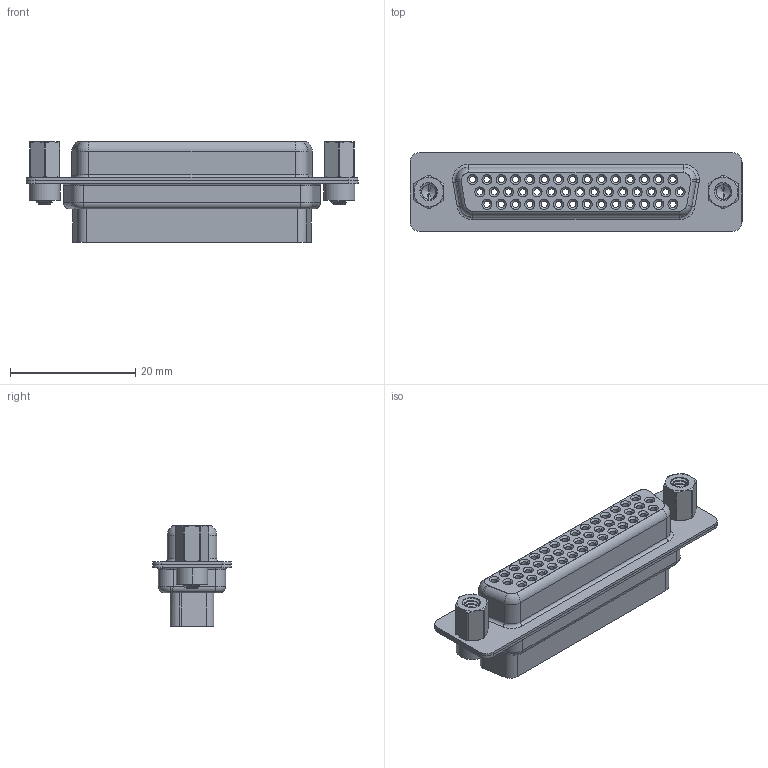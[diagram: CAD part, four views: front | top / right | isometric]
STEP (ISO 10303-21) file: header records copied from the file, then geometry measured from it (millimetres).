
FILE_DESCRIPTION (( 'STEP AP203' ), '1' );
FILE_NAME ('638-044-010-043.STEP', '2020-07-18T16:41:01', ( '' ), ( '' ), 'SwSTEP 2.0', 'SolidWorks 2020', '' );
FILE_SCHEMA (( 'CONFIG_CONTROL_DESIGN' ));
Length unit declared in the file: millimetre
Products named in the file (6): 638-044-010-043; 638 Housing_44 Contacts HP; 638 Shell Rear_44 Contacts; 638 Shell Front_44 Contacts; 638 4-40 Threaded Rivet; 638 4-40 Hex Standoff
Assembly tree (7 placements, depth 2):
  638-044-010-043
    638 Housing_44 Contacts HP
    638 Shell Front_44 Contacts
    638 Shell Rear_44 Contacts
    638 4-40 Threaded Rivet  x2
    638 4-40 Hex Standoff  x2
Bounding box: 53.04 x 12.6 x 16.1 mm (x, y, z)
Volume: 3690.5 mm3; surface area: 10024.2 mm2
Topology: 7 solids, 7 shells, 977 faces, 2265 edges, 1445 vertices
Faces by surface type: cylinder 561, plane 221, cone 120, torus 57, bspline 18
Entity records: 30079 total; most frequent: CARTESIAN_POINT 8724, DIRECTION 4705, ORIENTED_EDGE 4016, EDGE_CURVE 2008, AXIS2_PLACEMENT_3D 1983, VERTEX_POINT 1280, EDGE_LOOP 1126, CIRCLE 1101
